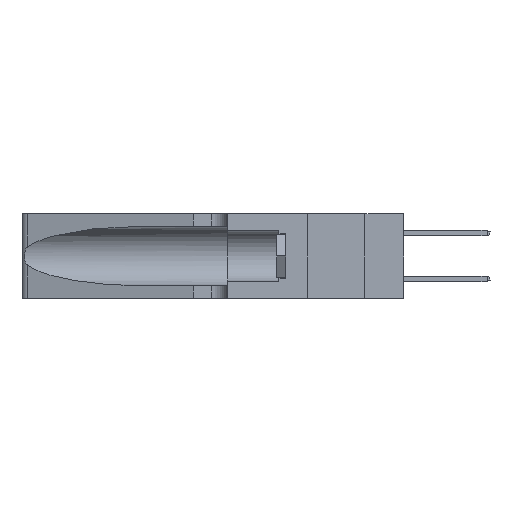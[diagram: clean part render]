
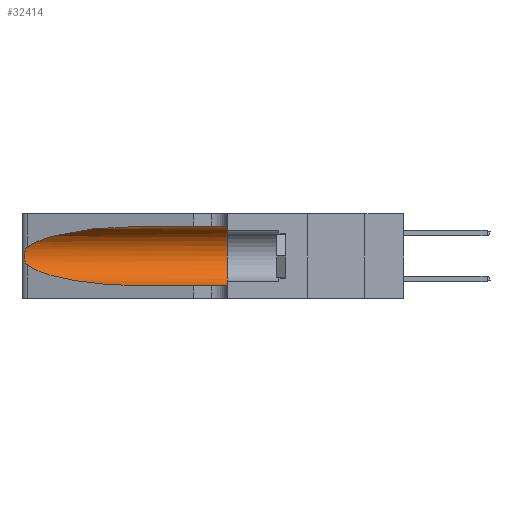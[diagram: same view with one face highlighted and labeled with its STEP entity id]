
A CAD part, left-side view. The second image highlights one B-rep face of the part: STEP entity #32414.
In plain terms, the highlighted cylindrical face has radius 3.308 mm (diameter 6.617 mm), a partial arc.
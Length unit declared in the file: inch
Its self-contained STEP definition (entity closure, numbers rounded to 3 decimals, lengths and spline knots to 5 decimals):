
#777 = CYLINDRICAL_SURFACE ( 'NONE', #5723, 0.13025 ) ;
#2402 = CARTESIAN_POINT ( 'NONE',  ( 0.26075, 1.23896, 0.19203 ) ) ;
#2974 = CARTESIAN_POINT ( 'NONE',  ( 0.1305, 0.35, 0.05475 ) ) ;
#2979 = FACE_OUTER_BOUND ( 'NONE', #44596, .T. ) ;
#3436 = B_SPLINE_CURVE_WITH_KNOTS ( 'NONE', 3,
 ( #33717, #44653, #9655, #12741, #34320, #37414, #2402, #12602, #13213, #16286, #37871, #30171, #40944, #19856 ),
 .UNSPECIFIED., .F., .F.,
 ( 4, 2, 2, 2, 2, 2, 4 ),
 ( 0., 0.00027, 0.00053, 0.00107, 0.0016, 0.00187, 0.00214 ),
 .UNSPECIFIED. ) ;
#4086 = ORIENTED_EDGE ( 'NONE', *, *, #39062, .F. ) ;
#4803 = CARTESIAN_POINT ( 'NONE',  ( 0.25487, 1.22718, 0.22369 ) ) ;
#5723 = AXIS2_PLACEMENT_3D ( 'NONE', #43428, #7997, #15996 ) ;
#5831 = DIRECTION ( 'NONE',  ( 0., -1., 0. ) ) ;
#5883 = CARTESIAN_POINT ( 'NONE',  ( 0.2373, 1.15595, 0.08982 ) ) ;
#6173 = EDGE_CURVE ( 'NONE', #34750, #8870, #45606, .T. ) ;
#6189 = CARTESIAN_POINT ( 'NONE',  ( 0.1305, 0.72297, 0.05475 ) ) ;
#7379 = DIRECTION ( 'NONE',  ( 0., 1., 0. ) ) ;
#7997 = DIRECTION ( 'NONE',  ( 0., -1., 0. ) ) ;
#8054 = CARTESIAN_POINT ( 'NONE',  ( 0.2373, 1.15595, 0.28018 ) ) ;
#8343 = ORIENTED_EDGE ( 'NONE', *, *, #20096, .T. ) ;
#8870 = VERTEX_POINT ( 'NONE', #2974 ) ;
#9119 = CARTESIAN_POINT ( 'NONE',  ( 0.25487, 1.22718, 0.22369 ) ) ;
#9540 = VERTEX_POINT ( 'NONE', #35633 ) ;
#9655 = CARTESIAN_POINT ( 'NONE',  ( 0.25639, 1.23184, 0.21858 ) ) ;
#10084 = CARTESIAN_POINT ( 'NONE',  ( 0.25487, 1.22718, 0.14631 ) ) ;
#10265 = VERTEX_POINT ( 'NONE', #11526 ) ;
#11526 = CARTESIAN_POINT ( 'NONE',  ( 0.1305, 0.72297, 0.31525 ) ) ;
#12602 = CARTESIAN_POINT ( 'NONE',  ( 0.26075, 1.23896, 0.178 ) ) ;
#12741 = CARTESIAN_POINT ( 'NONE',  ( 0.25787, 1.23484, 0.2124 ) ) ;
#13213 = CARTESIAN_POINT ( 'NONE',  ( 0.26017, 1.23833, 0.17102 ) ) ;
#15230 = ORIENTED_EDGE ( 'NONE', *, *, #21913, .T. ) ;
#15290 = CARTESIAN_POINT ( 'NONE',  ( 0.1305, 0.72297, 0.31525 ) ) ;
#15996 = DIRECTION ( 'NONE',  ( 0., 0., -1. ) ) ;
#16286 = CARTESIAN_POINT ( 'NONE',  ( 0.25856, 1.23593, 0.16098 ) ) ;
#16483 = DIRECTION ( 'NONE',  ( 0., -1., 0. ) ) ;
#16602 = EDGE_CURVE ( 'NONE', #41641, #9540, #36246, .T. ) ;
#18505 = LINE ( 'NONE', #30806, #40565 ) ;
#19856 = CARTESIAN_POINT ( 'NONE',  ( 0.25487, 1.22718, 0.14631 ) ) ;
#20096 = EDGE_CURVE ( 'NONE', #10265, #34113, #30024, .T. ) ;
#21913 = EDGE_CURVE ( 'NONE', #34113, #41641, #3436, .T. ) ;
#24052 = CARTESIAN_POINT ( 'NONE',  ( 0.18966, 0.96281, 0.05475 ) ) ;
#25257 = CARTESIAN_POINT ( 'NONE',  ( 0.1305, 0.35, 0.185 ) ) ;
#29407 = AXIS2_PLACEMENT_3D ( 'NONE', #25257, #7379, #42813 ) ;
#30024 =( BOUNDED_CURVE ( )  B_SPLINE_CURVE ( 3, ( #15290, #36573, #8054, #4803 ),
 .UNSPECIFIED., .F., .F. ) 
 B_SPLINE_CURVE_WITH_KNOTS ( ( 4, 4 ),
 ( 1.5708, 2.84003 ),
 .UNSPECIFIED. ) 
 CURVE ( )  GEOMETRIC_REPRESENTATION_ITEM ( )  RATIONAL_B_SPLINE_CURVE ( ( 1., 0.87, 0.87, 1. ) ) 
 REPRESENTATION_ITEM ( '' )  );
#30171 = CARTESIAN_POINT ( 'NONE',  ( 0.25639, 1.23186, 0.15144 ) ) ;
#30806 = CARTESIAN_POINT ( 'NONE',  ( 0.1305, 1.61858, 0.05475 ) ) ;
#32414 = ADVANCED_FACE ( 'NONE', ( #2979 ), #777, .F. ) ;
#33717 = CARTESIAN_POINT ( 'NONE',  ( 0.25487, 1.22718, 0.22369 ) ) ;
#34113 = VERTEX_POINT ( 'NONE', #9119 ) ;
#34320 = CARTESIAN_POINT ( 'NONE',  ( 0.25854, 1.2359, 0.20912 ) ) ;
#34334 = ORIENTED_EDGE ( 'NONE', *, *, #42791, .T. ) ;
#34750 = VERTEX_POINT ( 'NONE', #40378 ) ;
#35125 = LINE ( 'NONE', #37464, #43958 ) ;
#35353 = ORIENTED_EDGE ( 'NONE', *, *, #16602, .T. ) ;
#35633 = CARTESIAN_POINT ( 'NONE',  ( 0.1305, 0.72297, 0.05475 ) ) ;
#36246 =( BOUNDED_CURVE ( )  B_SPLINE_CURVE ( 3, ( #45190, #5883, #24052, #6189 ),
 .UNSPECIFIED., .F., .F. ) 
 B_SPLINE_CURVE_WITH_KNOTS ( ( 4, 4 ),
 ( 3.44316, 4.71239 ),
 .UNSPECIFIED. ) 
 CURVE ( )  GEOMETRIC_REPRESENTATION_ITEM ( )  RATIONAL_B_SPLINE_CURVE ( ( 1., 0.87, 0.87, 1. ) ) 
 REPRESENTATION_ITEM ( '' )  );
#36573 = CARTESIAN_POINT ( 'NONE',  ( 0.18966, 0.96281, 0.31525 ) ) ;
#37414 = CARTESIAN_POINT ( 'NONE',  ( 0.26018, 1.23835, 0.19895 ) ) ;
#37464 = CARTESIAN_POINT ( 'NONE',  ( 0.1305, 1.61858, 0.31525 ) ) ;
#37871 = CARTESIAN_POINT ( 'NONE',  ( 0.25789, 1.23486, 0.15765 ) ) ;
#39062 = EDGE_CURVE ( 'NONE', #10265, #34750, #35125, .T. ) ;
#40378 = CARTESIAN_POINT ( 'NONE',  ( 0.1305, 0.35, 0.31525 ) ) ;
#40565 = VECTOR ( 'NONE', #5831, 39.37008 ) ;
#40944 = CARTESIAN_POINT ( 'NONE',  ( 0.25555, 1.22993, 0.14849 ) ) ;
#40974 = ORIENTED_EDGE ( 'NONE', *, *, #6173, .F. ) ;
#41641 = VERTEX_POINT ( 'NONE', #10084 ) ;
#42791 = EDGE_CURVE ( 'NONE', #9540, #8870, #18505, .T. ) ;
#42813 = DIRECTION ( 'NONE',  ( 0., 0., 1. ) ) ;
#43428 = CARTESIAN_POINT ( 'NONE',  ( 0.1305, 1.61858, 0.185 ) ) ;
#43958 = VECTOR ( 'NONE', #16483, 39.37008 ) ;
#44596 = EDGE_LOOP ( 'NONE', ( #8343, #15230, #35353, #34334, #40974, #4086 ) ) ;
#44653 = CARTESIAN_POINT ( 'NONE',  ( 0.25555, 1.22994, 0.2215 ) ) ;
#45190 = CARTESIAN_POINT ( 'NONE',  ( 0.25487, 1.22718, 0.14631 ) ) ;
#45606 = CIRCLE ( 'NONE', #29407, 0.13025 ) ;
